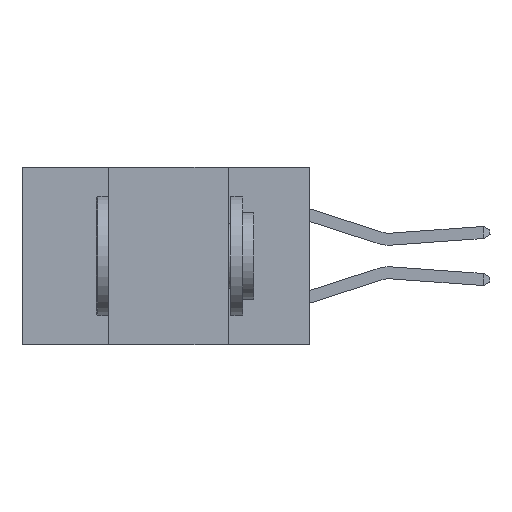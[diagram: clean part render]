
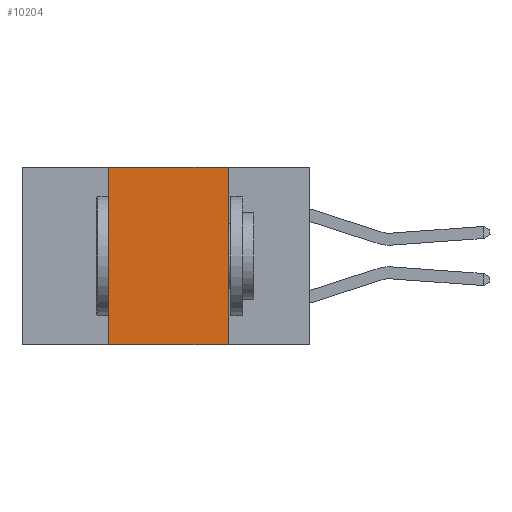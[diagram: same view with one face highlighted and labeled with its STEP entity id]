
A CAD part, left-side view. The second image highlights one B-rep face of the part: STEP entity #10204.
In plain terms, the highlighted planar face has unit normal (-1, 0, 0).
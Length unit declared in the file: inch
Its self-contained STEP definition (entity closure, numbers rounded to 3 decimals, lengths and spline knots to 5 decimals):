
#576 = VECTOR ( 'NONE', #10238, 39.37008 ) ;
#1364 = EDGE_CURVE ( 'NONE', #8178, #15387, #3138, .T. ) ;
#1814 = CARTESIAN_POINT ( 'NONE',  ( 0., 0.6, -0.37 ) ) ;
#1944 = CARTESIAN_POINT ( 'NONE',  ( 0., 0.17, -0.37 ) ) ;
#2026 = EDGE_CURVE ( 'NONE', #15387, #5205, #2527, .T. ) ;
#2527 = LINE ( 'NONE', #3749, #12337 ) ;
#2942 = EDGE_LOOP ( 'NONE', ( #11911, #5708, #7305, #9535 ) ) ;
#3138 = LINE ( 'NONE', #9583, #4013 ) ;
#3314 = CARTESIAN_POINT ( 'NONE',  ( 0., 0.42, -0.37 ) ) ;
#3749 = CARTESIAN_POINT ( 'NONE',  ( 0., 0.17, -0.37 ) ) ;
#4013 = VECTOR ( 'NONE', #10582, 39.37008 ) ;
#4780 = DIRECTION ( 'NONE',  ( 0., 0., -1. ) ) ;
#4970 = DIRECTION ( 'NONE',  ( 0., 0., -1. ) ) ;
#5061 = CARTESIAN_POINT ( 'NONE',  ( 0., 0.42, 0. ) ) ;
#5205 = VERTEX_POINT ( 'NONE', #1944 ) ;
#5457 = DIRECTION ( 'NONE',  ( 0., 0., 1. ) ) ;
#5708 = ORIENTED_EDGE ( 'NONE', *, *, #1364, .F. ) ;
#5932 = CARTESIAN_POINT ( 'NONE',  ( 0., 0.6, 0. ) ) ;
#6196 = EDGE_CURVE ( 'NONE', #14637, #8178, #10287, .T. ) ;
#6699 = CARTESIAN_POINT ( 'NONE',  ( 0., 0.42, -0.37 ) ) ;
#7069 = AXIS2_PLACEMENT_3D ( 'NONE', #5932, #10894, #4780 ) ;
#7151 = FACE_OUTER_BOUND ( 'NONE', #2942, .T. ) ;
#7305 = ORIENTED_EDGE ( 'NONE', *, *, #6196, .F. ) ;
#7891 = CARTESIAN_POINT ( 'NONE',  ( 0., 0.17, 0. ) ) ;
#8178 = VERTEX_POINT ( 'NONE', #5061 ) ;
#9535 = ORIENTED_EDGE ( 'NONE', *, *, #10705, .T. ) ;
#9583 = CARTESIAN_POINT ( 'NONE',  ( 0., 0.6, 0. ) ) ;
#10204 = ADVANCED_FACE ( 'NONE', ( #7151 ), #12121, .F. ) ;
#10238 = DIRECTION ( 'NONE',  ( 0., -1., 0. ) ) ;
#10287 = LINE ( 'NONE', #6699, #13791 ) ;
#10582 = DIRECTION ( 'NONE',  ( 0., -1., 0. ) ) ;
#10705 = EDGE_CURVE ( 'NONE', #14637, #5205, #14137, .T. ) ;
#10894 = DIRECTION ( 'NONE',  ( 1., 0., 0. ) ) ;
#11911 = ORIENTED_EDGE ( 'NONE', *, *, #2026, .F. ) ;
#12121 = PLANE ( 'NONE',  #7069 ) ;
#12337 = VECTOR ( 'NONE', #4970, 39.37008 ) ;
#13791 = VECTOR ( 'NONE', #5457, 39.37008 ) ;
#14137 = LINE ( 'NONE', #1814, #576 ) ;
#14637 = VERTEX_POINT ( 'NONE', #3314 ) ;
#15387 = VERTEX_POINT ( 'NONE', #7891 ) ;
